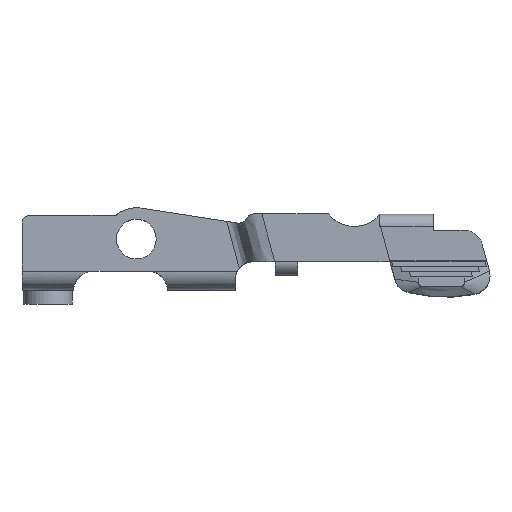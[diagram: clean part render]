
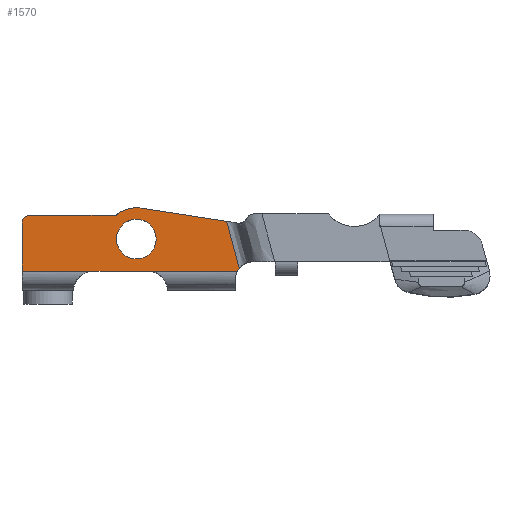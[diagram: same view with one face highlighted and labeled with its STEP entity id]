
A CAD part, top view. The second image highlights one B-rep face of the part: STEP entity #1570.
In plain terms, the highlighted planar face has unit normal (0, 0, 1).
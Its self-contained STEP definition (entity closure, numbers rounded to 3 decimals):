
#66 = CARTESIAN_POINT ( 'NONE',  ( 20.116, 8.875, 6.052 ) ) ;
#89 = VERTEX_POINT ( 'NONE', #175 ) ;
#175 = CARTESIAN_POINT ( 'NONE',  ( 32.648, 1.194, 6.052 ) ) ;
#304 = DIRECTION ( 'NONE',  ( -1., 0., 0. ) ) ;
#347 = CARTESIAN_POINT ( 'NONE',  ( 4.929, 7.969, 6.052 ) ) ;
#408 = LINE ( 'NONE', #2972, #5509 ) ;
#459 = DIRECTION ( 'NONE',  ( -0.707, 0.707, 0. ) ) ;
#554 = ORIENTED_EDGE ( 'NONE', *, *, #4815, .T. ) ;
#577 = AXIS2_PLACEMENT_3D ( 'NONE', #5596, #2642, #6097 ) ;
#604 = VERTEX_POINT ( 'NONE', #748 ) ;
#660 = LINE ( 'NONE', #2144, #4319 ) ;
#748 = CARTESIAN_POINT ( 'NONE',  ( 19.509, 8.922, 6.052 ) ) ;
#855 = AXIS2_PLACEMENT_3D ( 'NONE', #5194, #6192, #3239 ) ;
#857 = ORIENTED_EDGE ( 'NONE', *, *, #988, .F. ) ;
#859 = AXIS2_PLACEMENT_3D ( 'NONE', #1906, #5353, #2411 ) ;
#968 = ORIENTED_EDGE ( 'NONE', *, *, #4752, .T. ) ;
#988 = EDGE_CURVE ( 'NONE', #4901, #3196, #6287, .T. ) ;
#999 = DIRECTION ( 'NONE',  ( -0.988, 0.152, 0. ) ) ;
#1004 = ORIENTED_EDGE ( 'NONE', *, *, #3339, .T. ) ;
#1055 = VECTOR ( 'NONE', #304, 1000. ) ;
#1136 = CARTESIAN_POINT ( 'NONE',  ( 13.984, 0.845, 6.052 ) ) ;
#1319 = CIRCLE ( 'NONE', #2650, 3.988 ) ;
#1413 = CARTESIAN_POINT ( 'NONE',  ( 12.154, 0.845, 6.052 ) ) ;
#1570 = ADVANCED_FACE ( 'NONE', ( #3935, #5252 ), #5695, .T. ) ;
#1638 = DIRECTION ( 'NONE',  ( 1., 0., 0. ) ) ;
#1665 = DIRECTION ( 'NONE',  ( 0., 0., 1. ) ) ;
#1713 = CARTESIAN_POINT ( 'NONE',  ( 4.929, 6.953, 6.052 ) ) ;
#1796 = ORIENTED_EDGE ( 'NONE', *, *, #6247, .T. ) ;
#1856 = LINE ( 'NONE', #4533, #4324 ) ;
#1906 = CARTESIAN_POINT ( 'NONE',  ( 5.945, 6.953, 6.052 ) ) ;
#1949 = ORIENTED_EDGE ( 'NONE', *, *, #2950, .T. ) ;
#2144 = CARTESIAN_POINT ( 'NONE',  ( 13.984, 0.845, 6.052 ) ) ;
#2166 = CIRCLE ( 'NONE', #2803, 2.54 ) ;
#2246 = VECTOR ( 'NONE', #6348, 1000. ) ;
#2248 = CARTESIAN_POINT ( 'NONE',  ( 19.509, 4.934, 6.052 ) ) ;
#2281 = CARTESIAN_POINT ( 'NONE',  ( 19.509, 4.934, 6.052 ) ) ;
#2366 = EDGE_CURVE ( 'NONE', #5413, #5495, #2407, .T. ) ;
#2407 = LINE ( 'NONE', #1413, #2246 ) ;
#2411 = DIRECTION ( 'NONE',  ( -0.707, 0.707, 0. ) ) ;
#2494 = DIRECTION ( 'NONE',  ( -1., 0., 0. ) ) ;
#2511 = ORIENTED_EDGE ( 'NONE', *, *, #4958, .T. ) ;
#2553 = DIRECTION ( 'NONE',  ( 0., 0., -1. ) ) ;
#2557 = CARTESIAN_POINT ( 'NONE',  ( 16.922, 7.969, 6.052 ) ) ;
#2592 = ORIENTED_EDGE ( 'NONE', *, *, #3753, .F. ) ;
#2640 = EDGE_CURVE ( 'NONE', #2690, #4667, #6084, .T. ) ;
#2642 = DIRECTION ( 'NONE',  ( 0., 0., 1. ) ) ;
#2645 = EDGE_LOOP ( 'NONE', ( #968, #2511 ) ) ;
#2650 = AXIS2_PLACEMENT_3D ( 'NONE', #2248, #5687, #2730 ) ;
#2690 = VERTEX_POINT ( 'NONE', #2557 ) ;
#2709 = ORIENTED_EDGE ( 'NONE', *, *, #2366, .F. ) ;
#2730 = DIRECTION ( 'NONE',  ( 0., -1., 0. ) ) ;
#2768 = DIRECTION ( 'NONE',  ( -1., 0., 0. ) ) ;
#2803 = AXIS2_PLACEMENT_3D ( 'NONE', #5497, #2553, #6006 ) ;
#2950 = EDGE_CURVE ( 'NONE', #604, #2690, #1319, .T. ) ;
#2972 = CARTESIAN_POINT ( 'NONE',  ( 20.16, 8.868, 6.052 ) ) ;
#3196 = VERTEX_POINT ( 'NONE', #5690 ) ;
#3211 = CARTESIAN_POINT ( 'NONE',  ( 32.41, 0.845, 6.052 ) ) ;
#3228 = VERTEX_POINT ( 'NONE', #3211 ) ;
#3239 = DIRECTION ( 'NONE',  ( 1., 0., 0. ) ) ;
#3322 = VERTEX_POINT ( 'NONE', #4793 ) ;
#3323 = CIRCLE ( 'NONE', #3785, 3.988 ) ;
#3324 = DIRECTION ( 'NONE',  ( 0., -1., 0. ) ) ;
#3339 = EDGE_CURVE ( 'NONE', #4901, #5495, #4158, .T. ) ;
#3369 = VERTEX_POINT ( 'NONE', #4830 ) ;
#3422 = DIRECTION ( 'NONE',  ( 0., 0., -1. ) ) ;
#3449 = AXIS2_PLACEMENT_3D ( 'NONE', #2281, #5722, #2768 ) ;
#3671 = CARTESIAN_POINT ( 'NONE',  ( 4.929, 0.845, 6.052 ) ) ;
#3714 = VERTEX_POINT ( 'NONE', #5990 ) ;
#3753 = EDGE_CURVE ( 'NONE', #3322, #89, #1856, .T. ) ;
#3761 = CARTESIAN_POINT ( 'NONE',  ( 21.425, 0.845, 6.052 ) ) ;
#3785 = AXIS2_PLACEMENT_3D ( 'NONE', #4611, #1665, #5110 ) ;
#3906 = ORIENTED_EDGE ( 'NONE', *, *, #6075, .F. ) ;
#3935 = FACE_OUTER_BOUND ( 'NONE', #4276, .T. ) ;
#3953 = ORIENTED_EDGE ( 'NONE', *, *, #5575, .F. ) ;
#3969 = CARTESIAN_POINT ( 'NONE',  ( 5.945, 7.969, 6.052 ) ) ;
#4094 = CARTESIAN_POINT ( 'NONE',  ( 22.049, 4.934, 6.052 ) ) ;
#4158 = LINE ( 'NONE', #347, #4863 ) ;
#4252 = VERTEX_POINT ( 'NONE', #66 ) ;
#4276 = EDGE_LOOP ( 'NONE', ( #857, #1004, #2709, #6061, #3953, #6356, #2592, #1796, #554, #1949, #6057, #3906 ) ) ;
#4307 = EDGE_CURVE ( 'NONE', #89, #3228, #4333, .T. ) ;
#4319 = VECTOR ( 'NONE', #1638, 1000. ) ;
#4324 = VECTOR ( 'NONE', #5032, 1000. ) ;
#4333 = CIRCLE ( 'NONE', #577, 2.381 ) ;
#4533 = CARTESIAN_POINT ( 'NONE',  ( 30.578, 8.922, 6.052 ) ) ;
#4611 = CARTESIAN_POINT ( 'NONE',  ( 19.509, 4.934, 6.052 ) ) ;
#4667 = VERTEX_POINT ( 'NONE', #3969 ) ;
#4752 = EDGE_CURVE ( 'NONE', #3714, #6349, #2166, .T. ) ;
#4793 = CARTESIAN_POINT ( 'NONE',  ( 31.041, 7.193, 6.052 ) ) ;
#4815 = EDGE_CURVE ( 'NONE', #4252, #604, #3323, .T. ) ;
#4830 = CARTESIAN_POINT ( 'NONE',  ( 21.02, 0.845, 6.052 ) ) ;
#4856 = LINE ( 'NONE', #3761, #1055 ) ;
#4863 = VECTOR ( 'NONE', #3324, 1000. ) ;
#4901 = VERTEX_POINT ( 'NONE', #1713 ) ;
#4931 = VECTOR ( 'NONE', #2494, 1000. ) ;
#4952 = CARTESIAN_POINT ( 'NONE',  ( 16.922, 7.969, 6.052 ) ) ;
#4958 = EDGE_CURVE ( 'NONE', #6349, #3714, #5008, .T. ) ;
#5008 = CIRCLE ( 'NONE', #3449, 2.54 ) ;
#5032 = DIRECTION ( 'NONE',  ( 0.259, -0.966, 0. ) ) ;
#5110 = DIRECTION ( 'NONE',  ( 0., -1., 0. ) ) ;
#5150 = CIRCLE ( 'NONE', #859, 1.016 ) ;
#5194 = CARTESIAN_POINT ( 'NONE',  ( 19.379, 3.498, 6.052 ) ) ;
#5252 = FACE_BOUND ( 'NONE', #2645, .T. ) ;
#5353 = DIRECTION ( 'NONE',  ( 0., 0., -1. ) ) ;
#5413 = VERTEX_POINT ( 'NONE', #1136 ) ;
#5420 = EDGE_CURVE ( 'NONE', #5413, #3369, #660, .T. ) ;
#5495 = VERTEX_POINT ( 'NONE', #3671 ) ;
#5497 = CARTESIAN_POINT ( 'NONE',  ( 19.509, 4.934, 6.052 ) ) ;
#5509 = VECTOR ( 'NONE', #999, 1000. ) ;
#5575 = EDGE_CURVE ( 'NONE', #3228, #3369, #4856, .T. ) ;
#5596 = CARTESIAN_POINT ( 'NONE',  ( 34.489, -0.318, 6.052 ) ) ;
#5687 = DIRECTION ( 'NONE',  ( 0., 0., 1. ) ) ;
#5690 = CARTESIAN_POINT ( 'NONE',  ( 5.227, 7.672, 6.052 ) ) ;
#5695 = PLANE ( 'NONE',  #855 ) ;
#5722 = DIRECTION ( 'NONE',  ( 0., 0., -1. ) ) ;
#5990 = CARTESIAN_POINT ( 'NONE',  ( 16.969, 4.934, 6.052 ) ) ;
#6006 = DIRECTION ( 'NONE',  ( -1., 0., 0. ) ) ;
#6057 = ORIENTED_EDGE ( 'NONE', *, *, #2640, .T. ) ;
#6061 = ORIENTED_EDGE ( 'NONE', *, *, #5420, .T. ) ;
#6075 = EDGE_CURVE ( 'NONE', #3196, #4667, #5150, .T. ) ;
#6084 = LINE ( 'NONE', #4952, #4931 ) ;
#6097 = DIRECTION ( 'NONE',  ( -0.707, 0.707, 0. ) ) ;
#6184 = AXIS2_PLACEMENT_3D ( 'NONE', #6378, #3422, #459 ) ;
#6192 = DIRECTION ( 'NONE',  ( 0., 0., 1. ) ) ;
#6247 = EDGE_CURVE ( 'NONE', #3322, #4252, #408, .T. ) ;
#6287 = CIRCLE ( 'NONE', #6184, 1.016 ) ;
#6348 = DIRECTION ( 'NONE',  ( -1., 0., 0. ) ) ;
#6349 = VERTEX_POINT ( 'NONE', #4094 ) ;
#6356 = ORIENTED_EDGE ( 'NONE', *, *, #4307, .F. ) ;
#6378 = CARTESIAN_POINT ( 'NONE',  ( 5.945, 6.953, 6.052 ) ) ;
